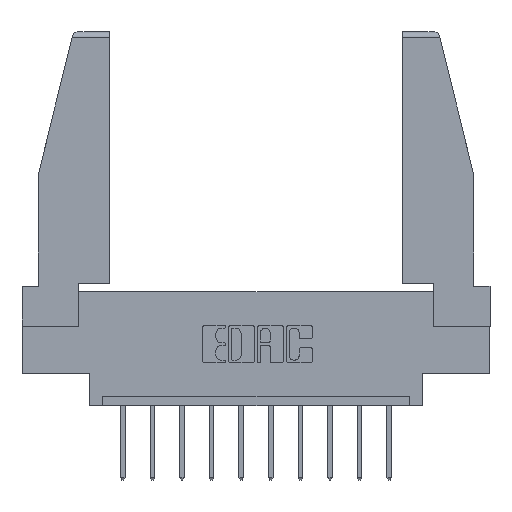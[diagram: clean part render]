
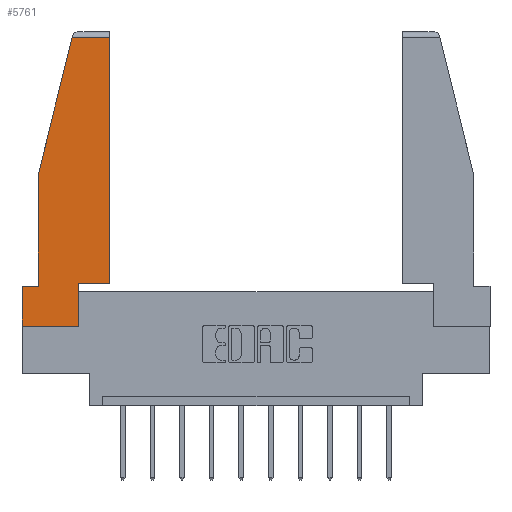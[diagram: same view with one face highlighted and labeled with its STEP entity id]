
A CAD part, top view. The second image highlights one B-rep face of the part: STEP entity #5761.
In plain terms, the highlighted planar face has unit normal (0, 0, 1).
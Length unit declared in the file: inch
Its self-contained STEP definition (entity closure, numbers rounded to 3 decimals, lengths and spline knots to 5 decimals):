
#989 = CARTESIAN_POINT ( 'NONE',  ( 0.297, 0.223, 0. ) ) ;
#1225 = VERTEX_POINT ( 'NONE', #2721 ) ;
#1326 = VECTOR ( 'NONE', #6551, 39.37008 ) ;
#1345 = VERTEX_POINT ( 'NONE', #2670 ) ;
#1364 = CARTESIAN_POINT ( 'NONE',  ( 0.086, 0.8, 0. ) ) ;
#1493 = CARTESIAN_POINT ( 'NONE',  ( 0.461, 1.52, 0. ) ) ;
#1794 = VERTEX_POINT ( 'NONE', #11847 ) ;
#1990 = DIRECTION ( 'NONE',  ( 0., 0., 1. ) ) ;
#2046 = DIRECTION ( 'NONE',  ( 0., 1., 0. ) ) ;
#2149 = EDGE_CURVE ( 'NONE', #1794, #11882, #4278, .T. ) ;
#2572 = ORIENTED_EDGE ( 'NONE', *, *, #11995, .T. ) ;
#2670 = CARTESIAN_POINT ( 'NONE',  ( 0.086, 0.8, 0. ) ) ;
#2721 = CARTESIAN_POINT ( 'NONE',  ( 0.297, 0., 0. ) ) ;
#2876 = VERTEX_POINT ( 'NONE', #12322 ) ;
#3236 = CARTESIAN_POINT ( 'NONE',  ( 0.297, 0., 0. ) ) ;
#3289 = CARTESIAN_POINT ( 'NONE',  ( 0.2636, 1.52, 0. ) ) ;
#3560 = DIRECTION ( 'NONE',  ( 0., -1., 0. ) ) ;
#3693 = EDGE_CURVE ( 'NONE', #1345, #10716, #8907, .T. ) ;
#3926 = LINE ( 'NONE', #10433, #13052 ) ;
#4198 = ORIENTED_EDGE ( 'NONE', *, *, #7139, .T. ) ;
#4278 = LINE ( 'NONE', #12956, #12543 ) ;
#4382 = VECTOR ( 'NONE', #12105, 39.37008 ) ;
#4976 = DIRECTION ( 'NONE',  ( 1., 0., 0. ) ) ;
#5018 = EDGE_LOOP ( 'NONE', ( #7360, #4198, #9499, #5376, #2572, #13076, #5019, #9013, #6322 ) ) ;
#5019 = ORIENTED_EDGE ( 'NONE', *, *, #8032, .T. ) ;
#5242 = VECTOR ( 'NONE', #6693, 39.37008 ) ;
#5268 = LINE ( 'NONE', #3236, #1326 ) ;
#5376 = ORIENTED_EDGE ( 'NONE', *, *, #3693, .T. ) ;
#5607 = CARTESIAN_POINT ( 'NONE',  ( 0.086, 0.21, 0. ) ) ;
#5633 = CARTESIAN_POINT ( 'NONE',  ( 0., 0., 0. ) ) ;
#5753 = VERTEX_POINT ( 'NONE', #989 ) ;
#5761 = ADVANCED_FACE ( 'NONE', ( #5980 ), #8636, .T. ) ;
#5980 = FACE_OUTER_BOUND ( 'NONE', #5018, .T. ) ;
#6121 = LINE ( 'NONE', #6585, #4382 ) ;
#6322 = ORIENTED_EDGE ( 'NONE', *, *, #8515, .T. ) ;
#6410 = CARTESIAN_POINT ( 'NONE',  ( 0., 0., 0. ) ) ;
#6551 = DIRECTION ( 'NONE',  ( 0., 1., 0. ) ) ;
#6585 = CARTESIAN_POINT ( 'NONE',  ( 0., 0.21, 0. ) ) ;
#6693 = DIRECTION ( 'NONE',  ( 1., 0., 0. ) ) ;
#7139 = EDGE_CURVE ( 'NONE', #11882, #11531, #8344, .T. ) ;
#7346 = DIRECTION ( 'NONE',  ( -1., 0., 0. ) ) ;
#7360 = ORIENTED_EDGE ( 'NONE', *, *, #2149, .T. ) ;
#7481 = DIRECTION ( 'NONE',  ( -1., 0., 0. ) ) ;
#7608 = CARTESIAN_POINT ( 'NONE',  ( 0., 0.21, 0. ) ) ;
#7647 = VECTOR ( 'NONE', #7481, 39.37008 ) ;
#7658 = AXIS2_PLACEMENT_3D ( 'NONE', #6410, #1990, #9792 ) ;
#8032 = EDGE_CURVE ( 'NONE', #2876, #1225, #10049, .T. ) ;
#8344 = LINE ( 'NONE', #12875, #7647 ) ;
#8515 = EDGE_CURVE ( 'NONE', #5753, #1794, #9746, .T. ) ;
#8636 = PLANE ( 'NONE',  #7658 ) ;
#8907 = LINE ( 'NONE', #1364, #9937 ) ;
#9013 = ORIENTED_EDGE ( 'NONE', *, *, #13378, .T. ) ;
#9056 = VECTOR ( 'NONE', #4976, 39.37008 ) ;
#9499 = ORIENTED_EDGE ( 'NONE', *, *, #12686, .T. ) ;
#9746 = LINE ( 'NONE', #10564, #9056 ) ;
#9792 = DIRECTION ( 'NONE',  ( 1., 0., 0. ) ) ;
#9937 = VECTOR ( 'NONE', #3560, 39.37008 ) ;
#10049 = LINE ( 'NONE', #5633, #5242 ) ;
#10433 = CARTESIAN_POINT ( 'NONE',  ( 0., 0.21, 0. ) ) ;
#10564 = CARTESIAN_POINT ( 'NONE',  ( 0.297, 0.223, 0. ) ) ;
#10694 = CARTESIAN_POINT ( 'NONE',  ( 0.271, 1.55, 0. ) ) ;
#10716 = VERTEX_POINT ( 'NONE', #5607 ) ;
#11531 = VERTEX_POINT ( 'NONE', #3289 ) ;
#11647 = DIRECTION ( 'NONE',  ( -0.239, -0.971, 0. ) ) ;
#11807 = VECTOR ( 'NONE', #11647, 39.37008 ) ;
#11847 = CARTESIAN_POINT ( 'NONE',  ( 0.461, 0.223, 0. ) ) ;
#11882 = VERTEX_POINT ( 'NONE', #1493 ) ;
#11995 = EDGE_CURVE ( 'NONE', #10716, #13419, #3926, .T. ) ;
#12105 = DIRECTION ( 'NONE',  ( 0., -1., 0. ) ) ;
#12322 = CARTESIAN_POINT ( 'NONE',  ( 0., 0., 0. ) ) ;
#12543 = VECTOR ( 'NONE', #2046, 39.37008 ) ;
#12686 = EDGE_CURVE ( 'NONE', #11531, #1345, #12702, .T. ) ;
#12702 = LINE ( 'NONE', #10694, #11807 ) ;
#12875 = CARTESIAN_POINT ( 'NONE',  ( 0., 1.52, 0. ) ) ;
#12956 = CARTESIAN_POINT ( 'NONE',  ( 0.461, 0.223, 0. ) ) ;
#13052 = VECTOR ( 'NONE', #7346, 39.37008 ) ;
#13076 = ORIENTED_EDGE ( 'NONE', *, *, #13999, .T. ) ;
#13378 = EDGE_CURVE ( 'NONE', #1225, #5753, #5268, .T. ) ;
#13419 = VERTEX_POINT ( 'NONE', #7608 ) ;
#13999 = EDGE_CURVE ( 'NONE', #13419, #2876, #6121, .T. ) ;
